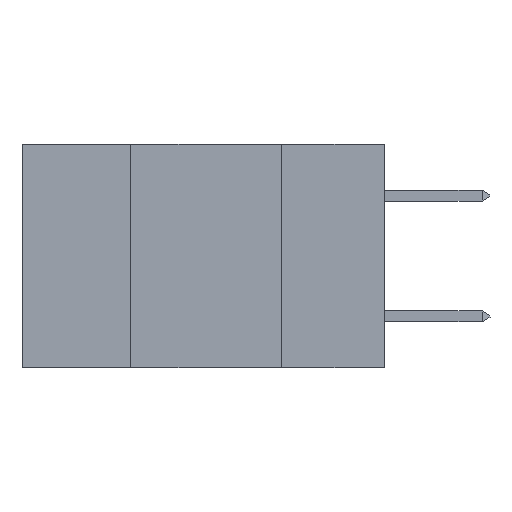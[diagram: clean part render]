
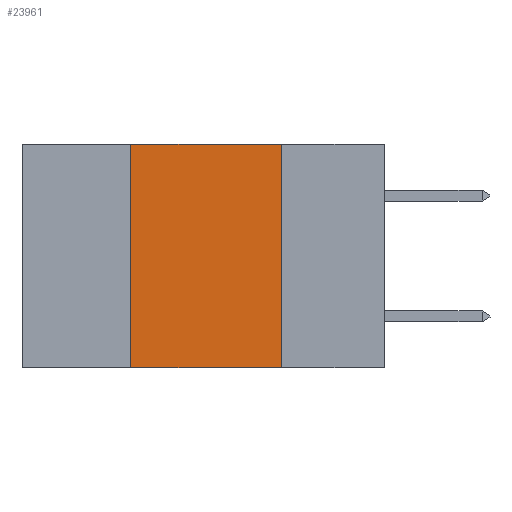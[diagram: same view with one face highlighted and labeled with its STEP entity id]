
A CAD part, left-side view. The second image highlights one B-rep face of the part: STEP entity #23961.
In plain terms, the highlighted planar face has unit normal (-1, 0, 0).
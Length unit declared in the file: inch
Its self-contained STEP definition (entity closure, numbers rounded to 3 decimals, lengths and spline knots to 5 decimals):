
#1676 = LINE ( 'NONE', #21867, #15974 ) ;
#3725 = VERTEX_POINT ( 'NONE', #22246 ) ;
#4541 = VECTOR ( 'NONE', #16190, 39.37008 ) ;
#5025 = CARTESIAN_POINT ( 'NONE',  ( 0., 0.17, 0. ) ) ;
#5151 = DIRECTION ( 'NONE',  ( 0., -1., 0. ) ) ;
#6572 = CARTESIAN_POINT ( 'NONE',  ( 0., 0.6, 0. ) ) ;
#7760 = EDGE_CURVE ( 'NONE', #10267, #11690, #20564, .T. ) ;
#8109 = ORIENTED_EDGE ( 'NONE', *, *, #10539, .T. ) ;
#9273 = ORIENTED_EDGE ( 'NONE', *, *, #24065, .F. ) ;
#9869 = CARTESIAN_POINT ( 'NONE',  ( 0., 0.42, 0. ) ) ;
#10267 = VERTEX_POINT ( 'NONE', #9869 ) ;
#10304 = DIRECTION ( 'NONE',  ( 1., 0., 0. ) ) ;
#10539 = EDGE_CURVE ( 'NONE', #18882, #3725, #1676, .T. ) ;
#10852 = DIRECTION ( 'NONE',  ( 0., 0., 1. ) ) ;
#11280 = ORIENTED_EDGE ( 'NONE', *, *, #7760, .F. ) ;
#11510 = CARTESIAN_POINT ( 'NONE',  ( 0., 0.42, -0.37 ) ) ;
#11690 = VERTEX_POINT ( 'NONE', #13870 ) ;
#13371 = ORIENTED_EDGE ( 'NONE', *, *, #15636, .F. ) ;
#13870 = CARTESIAN_POINT ( 'NONE',  ( 0., 0.17, 0. ) ) ;
#14440 = LINE ( 'NONE', #5025, #4541 ) ;
#15070 = AXIS2_PLACEMENT_3D ( 'NONE', #6572, #10304, #23362 ) ;
#15601 = VECTOR ( 'NONE', #20409, 39.37008 ) ;
#15636 = EDGE_CURVE ( 'NONE', #18882, #10267, #19256, .T. ) ;
#15873 = PLANE ( 'NONE',  #15070 ) ;
#15974 = VECTOR ( 'NONE', #5151, 39.37008 ) ;
#16190 = DIRECTION ( 'NONE',  ( 0., 0., -1. ) ) ;
#16661 = CARTESIAN_POINT ( 'NONE',  ( 0., 0.6, 0. ) ) ;
#18093 = VECTOR ( 'NONE', #10852, 39.37008 ) ;
#18302 = CARTESIAN_POINT ( 'NONE',  ( 0., 0.42, 0. ) ) ;
#18882 = VERTEX_POINT ( 'NONE', #11510 ) ;
#19256 = LINE ( 'NONE', #18302, #18093 ) ;
#20409 = DIRECTION ( 'NONE',  ( 0., -1., 0. ) ) ;
#20564 = LINE ( 'NONE', #16661, #15601 ) ;
#21867 = CARTESIAN_POINT ( 'NONE',  ( 0., 0.6, -0.37 ) ) ;
#22246 = CARTESIAN_POINT ( 'NONE',  ( 0., 0.17, -0.37 ) ) ;
#22320 = FACE_OUTER_BOUND ( 'NONE', #22358, .T. ) ;
#22358 = EDGE_LOOP ( 'NONE', ( #9273, #11280, #13371, #8109 ) ) ;
#23362 = DIRECTION ( 'NONE',  ( 0., 0., -1. ) ) ;
#23961 = ADVANCED_FACE ( 'NONE', ( #22320 ), #15873, .F. ) ;
#24065 = EDGE_CURVE ( 'NONE', #11690, #3725, #14440, .T. ) ;
